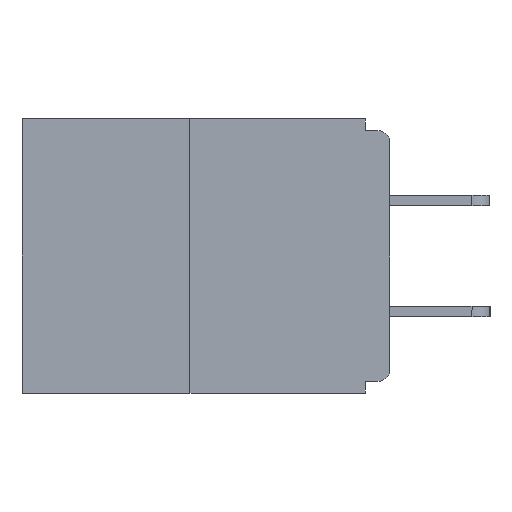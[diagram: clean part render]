
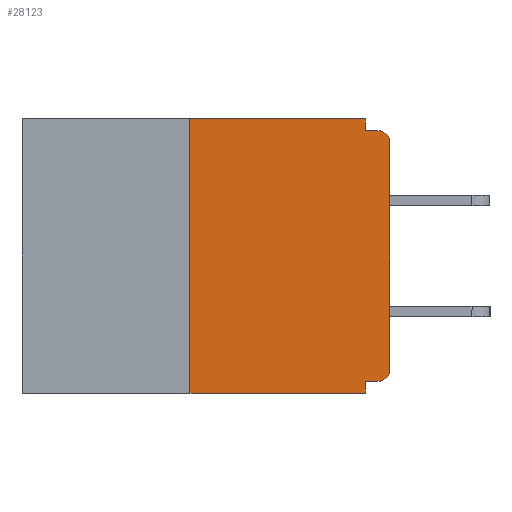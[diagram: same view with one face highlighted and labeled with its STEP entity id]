
A CAD part, left-side view. The second image highlights one B-rep face of the part: STEP entity #28123.
In plain terms, the highlighted planar face has unit normal (-1, 0, 0).
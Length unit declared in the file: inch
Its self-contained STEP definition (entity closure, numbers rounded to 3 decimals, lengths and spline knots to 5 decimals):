
#56 = LINE ( 'NONE', #2430, #7766 ) ;
#1043 = CARTESIAN_POINT ( 'NONE',  ( 0., 0.46, 0. ) ) ;
#2022 = VECTOR ( 'NONE', #20905, 39.37008 ) ;
#2430 = CARTESIAN_POINT ( 'NONE',  ( 0., 0.031, -0.343 ) ) ;
#2613 = ORIENTED_EDGE ( 'NONE', *, *, #3444, .T. ) ;
#2914 = CIRCLE ( 'NONE', #12853, 0.015 ) ;
#2971 = CARTESIAN_POINT ( 'NONE',  ( 0., 0., -0.313 ) ) ;
#2990 = LINE ( 'NONE', #6983, #20611 ) ;
#3166 = DIRECTION ( 'NONE',  ( 0., 0., -1. ) ) ;
#3298 = DIRECTION ( 'NONE',  ( 0., -1., 0. ) ) ;
#3340 = VECTOR ( 'NONE', #3298, 39.37008 ) ;
#3444 = EDGE_CURVE ( 'NONE', #13722, #10391, #11904, .T. ) ;
#4000 = VERTEX_POINT ( 'NONE', #14985 ) ;
#4152 = EDGE_CURVE ( 'NONE', #13722, #4000, #9792, .T. ) ;
#4262 = PLANE ( 'NONE',  #26737 ) ;
#4809 = FACE_OUTER_BOUND ( 'NONE', #27574, .T. ) ;
#4899 = ORIENTED_EDGE ( 'NONE', *, *, #27254, .F. ) ;
#5402 = LINE ( 'NONE', #12665, #13190 ) ;
#5690 = VERTEX_POINT ( 'NONE', #20429 ) ;
#5692 = CARTESIAN_POINT ( 'NONE',  ( 0., 0.015, -0.03 ) ) ;
#5899 = CARTESIAN_POINT ( 'NONE',  ( 0., 0.25, -0.343 ) ) ;
#6269 = ORIENTED_EDGE ( 'NONE', *, *, #25712, .F. ) ;
#6890 = EDGE_CURVE ( 'NONE', #7202, #29193, #2914, .T. ) ;
#6925 = VECTOR ( 'NONE', #22011, 39.37008 ) ;
#6932 = VECTOR ( 'NONE', #13002, 39.37008 ) ;
#6983 = CARTESIAN_POINT ( 'NONE',  ( 0., 0., -0.328 ) ) ;
#7202 = VERTEX_POINT ( 'NONE', #19429 ) ;
#7766 = VECTOR ( 'NONE', #18291, 39.37008 ) ;
#8466 = CARTESIAN_POINT ( 'NONE',  ( 0., 0.25, 0. ) ) ;
#8487 = ORIENTED_EDGE ( 'NONE', *, *, #17464, .T. ) ;
#8830 = VERTEX_POINT ( 'NONE', #23008 ) ;
#8876 = CARTESIAN_POINT ( 'NONE',  ( 0., 0.031, -0.015 ) ) ;
#8980 = CARTESIAN_POINT ( 'NONE',  ( 0., 0.031, -0.343 ) ) ;
#9025 = ORIENTED_EDGE ( 'NONE', *, *, #19822, .F. ) ;
#9157 = ORIENTED_EDGE ( 'NONE', *, *, #15724, .F. ) ;
#9792 = LINE ( 'NONE', #8466, #6932 ) ;
#10391 = VERTEX_POINT ( 'NONE', #8980 ) ;
#11037 = DIRECTION ( 'NONE',  ( 0., 0., -1. ) ) ;
#11207 = DIRECTION ( 'NONE',  ( 1., 0., 0. ) ) ;
#11904 = LINE ( 'NONE', #26153, #6925 ) ;
#12479 = ORIENTED_EDGE ( 'NONE', *, *, #24642, .T. ) ;
#12665 = CARTESIAN_POINT ( 'NONE',  ( 0., 0., 0. ) ) ;
#12837 = AXIS2_PLACEMENT_3D ( 'NONE', #5692, #28150, #3166 ) ;
#12853 = AXIS2_PLACEMENT_3D ( 'NONE', #21548, #24034, #23836 ) ;
#13002 = DIRECTION ( 'NONE',  ( 0., 0., 1. ) ) ;
#13190 = VECTOR ( 'NONE', #25804, 39.37008 ) ;
#13722 = VERTEX_POINT ( 'NONE', #5899 ) ;
#13994 = LINE ( 'NONE', #17941, #2022 ) ;
#14985 = CARTESIAN_POINT ( 'NONE',  ( 0., 0.25, 0. ) ) ;
#15724 = EDGE_CURVE ( 'NONE', #25673, #23870, #28829, .T. ) ;
#16050 = VECTOR ( 'NONE', #11037, 39.37008 ) ;
#16950 = ORIENTED_EDGE ( 'NONE', *, *, #26885, .F. ) ;
#17464 = EDGE_CURVE ( 'NONE', #29193, #17472, #5402, .T. ) ;
#17472 = VERTEX_POINT ( 'NONE', #23630 ) ;
#17941 = CARTESIAN_POINT ( 'NONE',  ( 0., 0., -0.015 ) ) ;
#18291 = DIRECTION ( 'NONE',  ( 0., 0., -1. ) ) ;
#19429 = CARTESIAN_POINT ( 'NONE',  ( 0., 0.015, -0.328 ) ) ;
#19822 = EDGE_CURVE ( 'NONE', #8830, #10391, #56, .T. ) ;
#20160 = CARTESIAN_POINT ( 'NONE',  ( 0., 0.46, 0. ) ) ;
#20429 = CARTESIAN_POINT ( 'NONE',  ( 0., 0.015, -0.015 ) ) ;
#20611 = VECTOR ( 'NONE', #27251, 39.37008 ) ;
#20905 = DIRECTION ( 'NONE',  ( 0., -1., 0. ) ) ;
#20966 = LINE ( 'NONE', #1043, #3340 ) ;
#21548 = CARTESIAN_POINT ( 'NONE',  ( 0., 0.015, -0.313 ) ) ;
#22011 = DIRECTION ( 'NONE',  ( 0., -1., 0. ) ) ;
#22589 = CARTESIAN_POINT ( 'NONE',  ( 0., 0.031, 0. ) ) ;
#23008 = CARTESIAN_POINT ( 'NONE',  ( 0., 0.031, -0.328 ) ) ;
#23630 = CARTESIAN_POINT ( 'NONE',  ( 0., 0., -0.03 ) ) ;
#23635 = ORIENTED_EDGE ( 'NONE', *, *, #4152, .F. ) ;
#23656 = ORIENTED_EDGE ( 'NONE', *, *, #6890, .T. ) ;
#23836 = DIRECTION ( 'NONE',  ( 0., 0., -1. ) ) ;
#23870 = VERTEX_POINT ( 'NONE', #8876 ) ;
#24034 = DIRECTION ( 'NONE',  ( -1., 0., 0. ) ) ;
#24642 = EDGE_CURVE ( 'NONE', #17472, #5690, #27228, .T. ) ;
#25478 = CARTESIAN_POINT ( 'NONE',  ( 0., 0.031, 0. ) ) ;
#25673 = VERTEX_POINT ( 'NONE', #25478 ) ;
#25712 = EDGE_CURVE ( 'NONE', #23870, #5690, #13994, .T. ) ;
#25804 = DIRECTION ( 'NONE',  ( 0., 0., 1. ) ) ;
#26153 = CARTESIAN_POINT ( 'NONE',  ( 0., 0.46, -0.343 ) ) ;
#26737 = AXIS2_PLACEMENT_3D ( 'NONE', #20160, #11207, #27006 ) ;
#26885 = EDGE_CURVE ( 'NONE', #4000, #25673, #20966, .T. ) ;
#27006 = DIRECTION ( 'NONE',  ( 0., 0., -1. ) ) ;
#27228 = CIRCLE ( 'NONE', #12837, 0.015 ) ;
#27251 = DIRECTION ( 'NONE',  ( 0., 1., 0. ) ) ;
#27254 = EDGE_CURVE ( 'NONE', #7202, #8830, #2990, .T. ) ;
#27574 = EDGE_LOOP ( 'NONE', ( #16950, #23635, #2613, #9025, #4899, #23656, #8487, #12479, #6269, #9157 ) ) ;
#28123 = ADVANCED_FACE ( 'NONE', ( #4809 ), #4262, .F. ) ;
#28150 = DIRECTION ( 'NONE',  ( -1., 0., 0. ) ) ;
#28829 = LINE ( 'NONE', #22589, #16050 ) ;
#29193 = VERTEX_POINT ( 'NONE', #2971 ) ;
